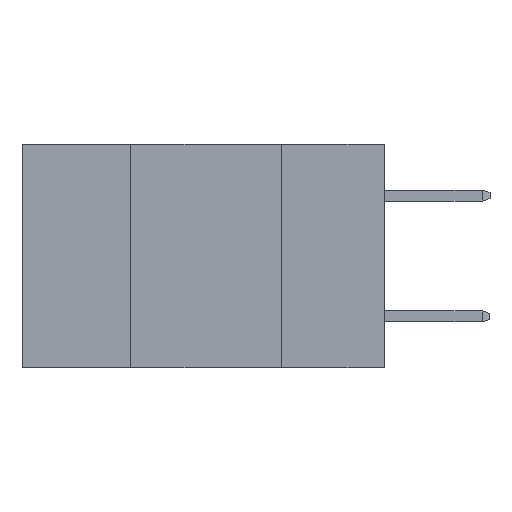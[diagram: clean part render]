
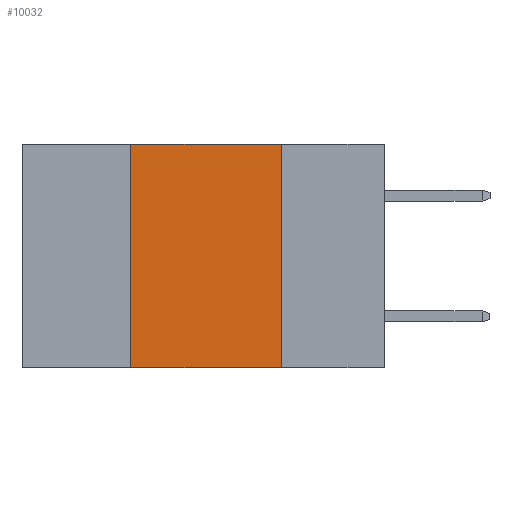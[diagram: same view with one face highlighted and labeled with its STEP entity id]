
A CAD part, left-side view. The second image highlights one B-rep face of the part: STEP entity #10032.
In plain terms, the highlighted planar face has unit normal (-1, 0, 0).
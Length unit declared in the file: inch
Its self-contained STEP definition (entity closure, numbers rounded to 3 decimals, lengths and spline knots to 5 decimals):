
#1069 = EDGE_LOOP ( 'NONE', ( #10024, #9168, #2365, #9418 ) ) ;
#1122 = VERTEX_POINT ( 'NONE', #4873 ) ;
#1308 = VERTEX_POINT ( 'NONE', #9744 ) ;
#1689 = PLANE ( 'NONE',  #6518 ) ;
#2077 = VECTOR ( 'NONE', #10389, 39.37008 ) ;
#2253 = LINE ( 'NONE', #4832, #10715 ) ;
#2352 = LINE ( 'NONE', #6357, #2077 ) ;
#2365 = ORIENTED_EDGE ( 'NONE', *, *, #7837, .F. ) ;
#2511 = EDGE_CURVE ( 'NONE', #3799, #7956, #9613, .T. ) ;
#3105 = EDGE_CURVE ( 'NONE', #1308, #1122, #6164, .T. ) ;
#3109 = CARTESIAN_POINT ( 'NONE',  ( 0., 0.17, 0. ) ) ;
#3425 = DIRECTION ( 'NONE',  ( 0., 0., -1. ) ) ;
#3444 = DIRECTION ( 'NONE',  ( 0., -1., 0. ) ) ;
#3799 = VERTEX_POINT ( 'NONE', #9213 ) ;
#4832 = CARTESIAN_POINT ( 'NONE',  ( 0., 0.17, 0. ) ) ;
#4873 = CARTESIAN_POINT ( 'NONE',  ( 0., 0.17, -0.37 ) ) ;
#6164 = LINE ( 'NONE', #7030, #8376 ) ;
#6357 = CARTESIAN_POINT ( 'NONE',  ( 0., 0.42, 0. ) ) ;
#6518 = AXIS2_PLACEMENT_3D ( 'NONE', #7622, #8444, #3425 ) ;
#6684 = EDGE_CURVE ( 'NONE', #7956, #1122, #2253, .T. ) ;
#7030 = CARTESIAN_POINT ( 'NONE',  ( 0., 0.6, -0.37 ) ) ;
#7209 = VECTOR ( 'NONE', #3444, 39.37008 ) ;
#7326 = DIRECTION ( 'NONE',  ( 0., -1., 0. ) ) ;
#7568 = FACE_OUTER_BOUND ( 'NONE', #1069, .T. ) ;
#7622 = CARTESIAN_POINT ( 'NONE',  ( 0., 0.6, 0. ) ) ;
#7837 = EDGE_CURVE ( 'NONE', #1308, #3799, #2352, .T. ) ;
#7956 = VERTEX_POINT ( 'NONE', #3109 ) ;
#8376 = VECTOR ( 'NONE', #7326, 39.37008 ) ;
#8444 = DIRECTION ( 'NONE',  ( 1., 0., 0. ) ) ;
#8678 = CARTESIAN_POINT ( 'NONE',  ( 0., 0.6, 0. ) ) ;
#8992 = DIRECTION ( 'NONE',  ( 0., 0., -1. ) ) ;
#9168 = ORIENTED_EDGE ( 'NONE', *, *, #2511, .F. ) ;
#9213 = CARTESIAN_POINT ( 'NONE',  ( 0., 0.42, 0. ) ) ;
#9418 = ORIENTED_EDGE ( 'NONE', *, *, #3105, .T. ) ;
#9613 = LINE ( 'NONE', #8678, #7209 ) ;
#9744 = CARTESIAN_POINT ( 'NONE',  ( 0., 0.42, -0.37 ) ) ;
#10024 = ORIENTED_EDGE ( 'NONE', *, *, #6684, .F. ) ;
#10032 = ADVANCED_FACE ( 'NONE', ( #7568 ), #1689, .F. ) ;
#10389 = DIRECTION ( 'NONE',  ( 0., 0., 1. ) ) ;
#10715 = VECTOR ( 'NONE', #8992, 39.37008 ) ;
